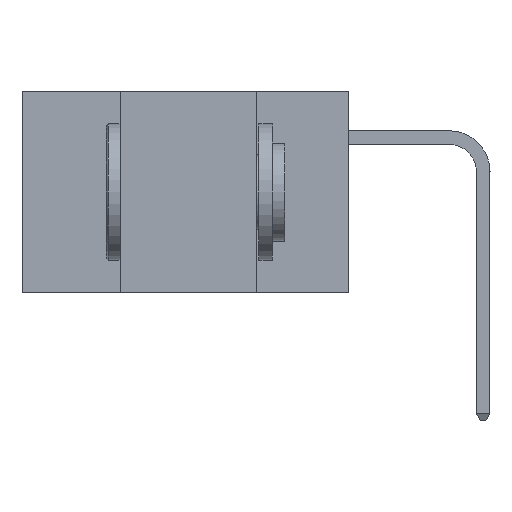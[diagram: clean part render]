
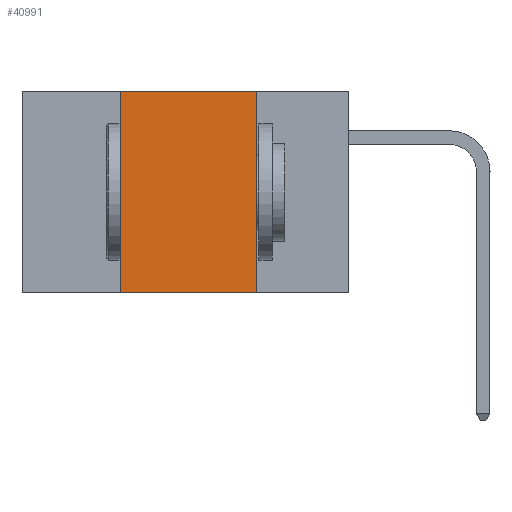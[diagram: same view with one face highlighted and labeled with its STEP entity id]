
A CAD part, left-side view. The second image highlights one B-rep face of the part: STEP entity #40991.
In plain terms, the highlighted planar face has unit normal (-1, 0, 0).
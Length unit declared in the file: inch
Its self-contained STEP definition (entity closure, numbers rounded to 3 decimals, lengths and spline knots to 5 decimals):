
#1440 = VERTEX_POINT ( 'NONE', #7654 ) ;
#2851 = FACE_OUTER_BOUND ( 'NONE', #25172, .T. ) ;
#3755 = PLANE ( 'NONE',  #18963 ) ;
#5483 = DIRECTION ( 'NONE',  ( 0., -1., 0. ) ) ;
#7149 = CARTESIAN_POINT ( 'NONE',  ( 0., 0.6, 0. ) ) ;
#7654 = CARTESIAN_POINT ( 'NONE',  ( 0., 0.42, 0. ) ) ;
#8573 = CARTESIAN_POINT ( 'NONE',  ( 0., 0.6, -0.37 ) ) ;
#8902 = CARTESIAN_POINT ( 'NONE',  ( 0., 0.42, 0. ) ) ;
#10396 = VECTOR ( 'NONE', #40160, 39.37008 ) ;
#12111 = CARTESIAN_POINT ( 'NONE',  ( 0., 0.17, 0. ) ) ;
#12162 = DIRECTION ( 'NONE',  ( 0., 0., 1. ) ) ;
#12211 = CARTESIAN_POINT ( 'NONE',  ( 0., 0.42, -0.37 ) ) ;
#12547 = ORIENTED_EDGE ( 'NONE', *, *, #22714, .F. ) ;
#13340 = EDGE_CURVE ( 'NONE', #1440, #13534, #22640, .T. ) ;
#13534 = VERTEX_POINT ( 'NONE', #12111 ) ;
#14987 = LINE ( 'NONE', #8902, #23504 ) ;
#16414 = CARTESIAN_POINT ( 'NONE',  ( 0., 0.17, 0. ) ) ;
#17013 = DIRECTION ( 'NONE',  ( 1., 0., 0. ) ) ;
#18963 = AXIS2_PLACEMENT_3D ( 'NONE', #7149, #17013, #39536 ) ;
#20976 = LINE ( 'NONE', #16414, #10396 ) ;
#21654 = VECTOR ( 'NONE', #37558, 39.37008 ) ;
#21960 = VERTEX_POINT ( 'NONE', #12211 ) ;
#22640 = LINE ( 'NONE', #41037, #21654 ) ;
#22714 = EDGE_CURVE ( 'NONE', #13534, #27214, #20976, .T. ) ;
#23138 = ORIENTED_EDGE ( 'NONE', *, *, #28051, .T. ) ;
#23504 = VECTOR ( 'NONE', #12162, 39.37008 ) ;
#25172 = EDGE_LOOP ( 'NONE', ( #12547, #25818, #29483, #23138 ) ) ;
#25818 = ORIENTED_EDGE ( 'NONE', *, *, #13340, .F. ) ;
#27214 = VERTEX_POINT ( 'NONE', #30182 ) ;
#28051 = EDGE_CURVE ( 'NONE', #21960, #27214, #39386, .T. ) ;
#29483 = ORIENTED_EDGE ( 'NONE', *, *, #30473, .F. ) ;
#30182 = CARTESIAN_POINT ( 'NONE',  ( 0., 0.17, -0.37 ) ) ;
#30473 = EDGE_CURVE ( 'NONE', #21960, #1440, #14987, .T. ) ;
#30869 = VECTOR ( 'NONE', #5483, 39.37008 ) ;
#37558 = DIRECTION ( 'NONE',  ( 0., -1., 0. ) ) ;
#39386 = LINE ( 'NONE', #8573, #30869 ) ;
#39536 = DIRECTION ( 'NONE',  ( 0., 0., -1. ) ) ;
#40160 = DIRECTION ( 'NONE',  ( 0., 0., -1. ) ) ;
#40991 = ADVANCED_FACE ( 'NONE', ( #2851 ), #3755, .F. ) ;
#41037 = CARTESIAN_POINT ( 'NONE',  ( 0., 0.6, 0. ) ) ;
